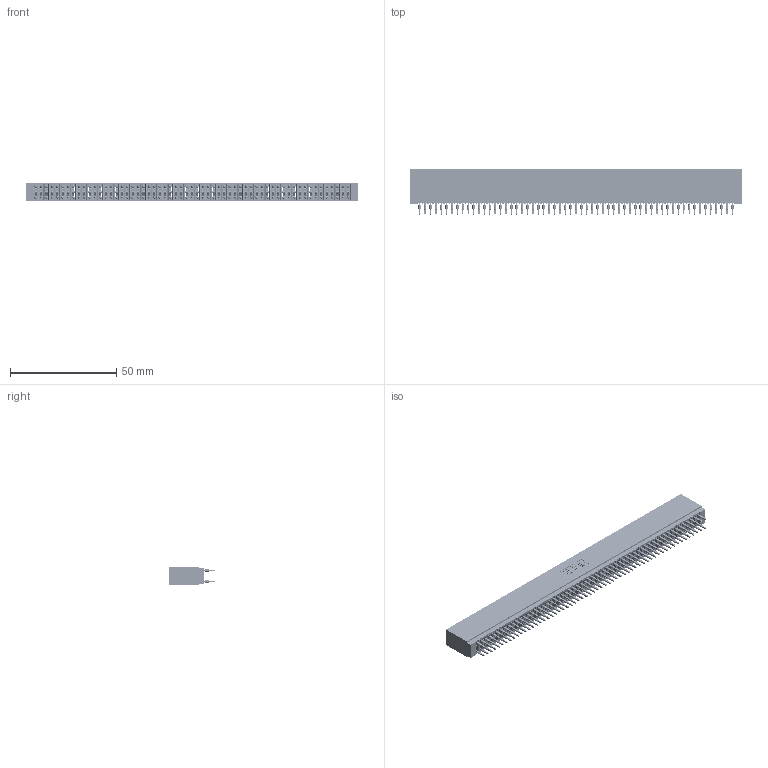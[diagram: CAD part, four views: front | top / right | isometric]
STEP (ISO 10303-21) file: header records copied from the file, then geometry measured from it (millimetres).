
FILE_DESCRIPTION (( 'STEP AP203' ), '1' );
FILE_NAME ('745-118-560-201.STEP', '2026-02-27T01:15:59', ( '' ), ( '' ), 'SwSTEP 2.0', 'SolidWorks 2023', '' );
FILE_SCHEMA (( 'CONFIG_CONTROL_DESIGN' ));
Length unit declared in the file: millimetre
Products named in the file (3): 745-118-560-201; 745 Part_Insulator Option - 01; 745-292-001_560
Assembly tree (119 placements, depth 2):
  745-118-560-201
    745 Part_Insulator Option - 01
    745-292-001_560  x118
Bounding box: 156.46 x 21.22 x 8.89 mm (x, y, z)
Volume: 14424.9 mm3; surface area: 31579 mm2
Topology: 119 solids, 119 shells, 11718 faces, 32059 edges, 20350 vertices
Faces by surface type: plane 6073, cylinder 2577, bspline 2360, torus 708
Entity records: 97330 total; most frequent: CARTESIAN_POINT 17381, ORIENTED_EDGE 16850, DIRECTION 14709, EDGE_CURVE 8425, LINE 7881, VECTOR 7881, VERTEX_POINT 5374, AXIS2_PLACEMENT_3D 3414
